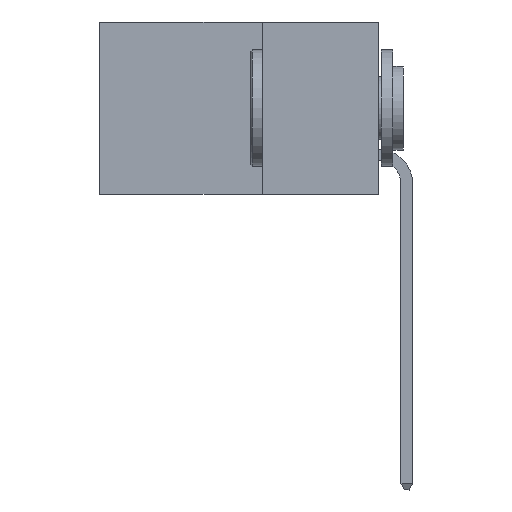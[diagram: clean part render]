
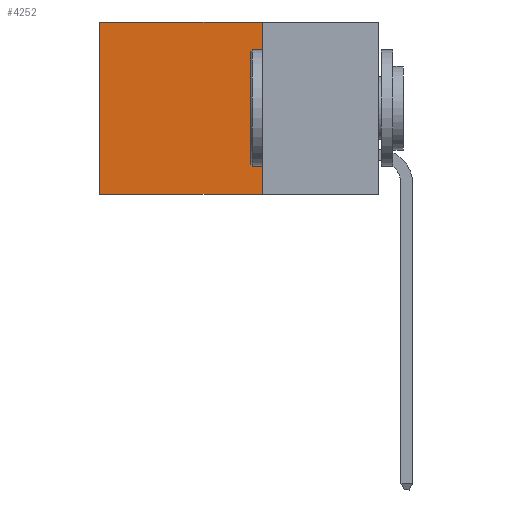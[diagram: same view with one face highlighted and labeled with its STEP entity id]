
A CAD part, left-side view. The second image highlights one B-rep face of the part: STEP entity #4252.
In plain terms, the highlighted planar face has unit normal (-1, 0, 0).
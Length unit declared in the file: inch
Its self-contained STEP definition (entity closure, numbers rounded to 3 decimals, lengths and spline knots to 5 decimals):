
#71 = EDGE_LOOP ( 'NONE', ( #5417, #22281, #12933, #13405 ) ) ;
#268 = EDGE_CURVE ( 'NONE', #14180, #18318, #11198, .T. ) ;
#295 = DIRECTION ( 'NONE',  ( 0., 1., 0. ) ) ;
#1167 = CARTESIAN_POINT ( 'NONE',  ( 0.298, 0.6, 0. ) ) ;
#2809 = EDGE_CURVE ( 'NONE', #3804, #18318, #2993, .T. ) ;
#2993 = LINE ( 'NONE', #20851, #14347 ) ;
#3632 = FACE_OUTER_BOUND ( 'NONE', #71, .T. ) ;
#3804 = VERTEX_POINT ( 'NONE', #15778 ) ;
#4252 = ADVANCED_FACE ( 'NONE', ( #3632 ), #4867, .F. ) ;
#4867 = PLANE ( 'NONE',  #10345 ) ;
#5417 = ORIENTED_EDGE ( 'NONE', *, *, #268, .T. ) ;
#5889 = LINE ( 'NONE', #6719, #10929 ) ;
#6053 = CARTESIAN_POINT ( 'NONE',  ( 0.298, 0.25, 0. ) ) ;
#6391 = EDGE_CURVE ( 'NONE', #20434, #3804, #18582, .T. ) ;
#6719 = CARTESIAN_POINT ( 'NONE',  ( 0.298, 0.25, 0. ) ) ;
#7905 = DIRECTION ( 'NONE',  ( 0., 0., -1. ) ) ;
#9258 = CARTESIAN_POINT ( 'NONE',  ( 0.298, 0.25, 0. ) ) ;
#9287 = DIRECTION ( 'NONE',  ( 1., 0., 0. ) ) ;
#10345 = AXIS2_PLACEMENT_3D ( 'NONE', #9258, #9287, #7905 ) ;
#10568 = CARTESIAN_POINT ( 'NONE',  ( 0.298, 0.6, -0.37 ) ) ;
#10929 = VECTOR ( 'NONE', #295, 39.37008 ) ;
#11198 = LINE ( 'NONE', #18641, #22587 ) ;
#12088 = EDGE_CURVE ( 'NONE', #20434, #14180, #5889, .T. ) ;
#12933 = ORIENTED_EDGE ( 'NONE', *, *, #6391, .F. ) ;
#13405 = ORIENTED_EDGE ( 'NONE', *, *, #12088, .T. ) ;
#13901 = DIRECTION ( 'NONE',  ( 0., 0., -1. ) ) ;
#14180 = VERTEX_POINT ( 'NONE', #1167 ) ;
#14347 = VECTOR ( 'NONE', #21109, 39.37008 ) ;
#15509 = VECTOR ( 'NONE', #13901, 39.37008 ) ;
#15778 = CARTESIAN_POINT ( 'NONE',  ( 0.298, 0.25, -0.37 ) ) ;
#16061 = CARTESIAN_POINT ( 'NONE',  ( 0.298, 0.25, 0. ) ) ;
#18318 = VERTEX_POINT ( 'NONE', #10568 ) ;
#18582 = LINE ( 'NONE', #16061, #15509 ) ;
#18641 = CARTESIAN_POINT ( 'NONE',  ( 0.298, 0.6, 0. ) ) ;
#20434 = VERTEX_POINT ( 'NONE', #6053 ) ;
#20851 = CARTESIAN_POINT ( 'NONE',  ( 0.298, 0.25, -0.37 ) ) ;
#21109 = DIRECTION ( 'NONE',  ( 0., 1., 0. ) ) ;
#22281 = ORIENTED_EDGE ( 'NONE', *, *, #2809, .F. ) ;
#22587 = VECTOR ( 'NONE', #24554, 39.37008 ) ;
#24554 = DIRECTION ( 'NONE',  ( 0., 0., -1. ) ) ;
